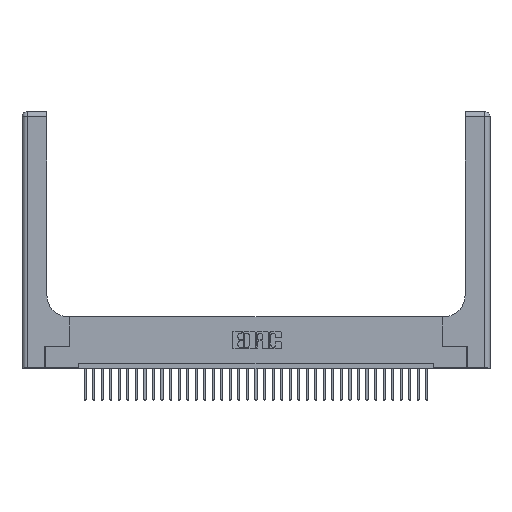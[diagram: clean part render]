
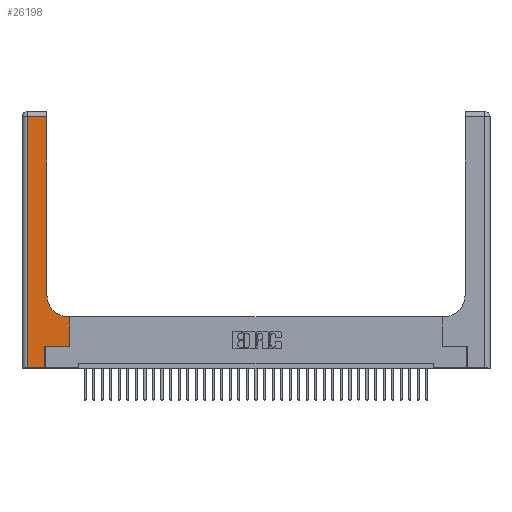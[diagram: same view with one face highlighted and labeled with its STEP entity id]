
A CAD part, top view. The second image highlights one B-rep face of the part: STEP entity #26198.
In plain terms, the highlighted planar face has unit normal (0, 0, 1).
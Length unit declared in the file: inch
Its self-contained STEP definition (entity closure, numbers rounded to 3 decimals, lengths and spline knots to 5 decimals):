
#583 = EDGE_CURVE ( 'NONE', #14601, #16200, #6018, .T. ) ;
#840 = CARTESIAN_POINT ( 'NONE',  ( 0.5585, 0.6, 0.37 ) ) ;
#1025 = DIRECTION ( 'NONE',  ( -1., 0., 0. ) ) ;
#1134 = CARTESIAN_POINT ( 'NONE',  ( 0.269, 0., 0.37 ) ) ;
#1947 = CIRCLE ( 'NONE', #6414, 0.25 ) ;
#1980 = LINE ( 'NONE', #19716, #35661 ) ;
#2318 = CARTESIAN_POINT ( 'NONE',  ( 0.06, 2.94, 0.37 ) ) ;
#2883 = DIRECTION ( 'NONE',  ( 1., 0., 0. ) ) ;
#3247 = ORIENTED_EDGE ( 'NONE', *, *, #31502, .T. ) ;
#3248 = VERTEX_POINT ( 'NONE', #18305 ) ;
#4439 = LINE ( 'NONE', #34091, #11006 ) ;
#4556 = DIRECTION ( 'NONE',  ( 1., 0., 0. ) ) ;
#5342 = VERTEX_POINT ( 'NONE', #9068 ) ;
#6018 = LINE ( 'NONE', #27974, #23095 ) ;
#6247 = EDGE_CURVE ( 'NONE', #16200, #3248, #16353, .T. ) ;
#6414 = AXIS2_PLACEMENT_3D ( 'NONE', #30180, #16047, #21751 ) ;
#6669 = CARTESIAN_POINT ( 'NONE',  ( 0.2915, 3., 0.37 ) ) ;
#7341 = LINE ( 'NONE', #6669, #21810 ) ;
#7647 = ORIENTED_EDGE ( 'NONE', *, *, #14574, .T. ) ;
#8733 = VERTEX_POINT ( 'NONE', #18860 ) ;
#9068 = CARTESIAN_POINT ( 'NONE',  ( 0.5415, 0.6, 0.37 ) ) ;
#9907 = ORIENTED_EDGE ( 'NONE', *, *, #32050, .T. ) ;
#10061 = CARTESIAN_POINT ( 'NONE',  ( 0.06, 3., 0.37 ) ) ;
#10184 = CARTESIAN_POINT ( 'NONE',  ( 0.269, 0.25, 0.37 ) ) ;
#10633 = CARTESIAN_POINT ( 'NONE',  ( 0.269, 0., 0.37 ) ) ;
#11006 = VECTOR ( 'NONE', #25754, 39.37008 ) ;
#11677 = CARTESIAN_POINT ( 'NONE',  ( 0.2915, 2.94, 0.37 ) ) ;
#11682 = EDGE_CURVE ( 'NONE', #3248, #31371, #22265, .T. ) ;
#12402 = LINE ( 'NONE', #17424, #30776 ) ;
#14312 = PLANE ( 'NONE',  #20672 ) ;
#14538 = VECTOR ( 'NONE', #27490, 39.37008 ) ;
#14574 = EDGE_CURVE ( 'NONE', #28070, #32074, #12402, .T. ) ;
#14601 = VERTEX_POINT ( 'NONE', #30248 ) ;
#16047 = DIRECTION ( 'NONE',  ( 0., 0., -1. ) ) ;
#16200 = VERTEX_POINT ( 'NONE', #1134 ) ;
#16353 = LINE ( 'NONE', #10633, #14538 ) ;
#17007 = CARTESIAN_POINT ( 'NONE',  ( 0., 3., 0.37 ) ) ;
#17248 = DIRECTION ( 'NONE',  ( 0., 0., -1. ) ) ;
#17424 = CARTESIAN_POINT ( 'NONE',  ( 0., 2.94, 0.37 ) ) ;
#18305 = CARTESIAN_POINT ( 'NONE',  ( 0.269, 0.25, 0.37 ) ) ;
#18860 = CARTESIAN_POINT ( 'NONE',  ( 0.2915, 0.85, 0.37 ) ) ;
#19140 = DIRECTION ( 'NONE',  ( 0., -1., 0. ) ) ;
#19222 = ORIENTED_EDGE ( 'NONE', *, *, #24231, .T. ) ;
#19716 = CARTESIAN_POINT ( 'NONE',  ( 0.5585, 0.25, 0.37 ) ) ;
#20672 = AXIS2_PLACEMENT_3D ( 'NONE', #17007, #17248, #33846 ) ;
#21419 = ORIENTED_EDGE ( 'NONE', *, *, #25837, .T. ) ;
#21751 = DIRECTION ( 'NONE',  ( 1., 0., 0. ) ) ;
#21810 = VECTOR ( 'NONE', #26244, 39.37008 ) ;
#22215 = LINE ( 'NONE', #10061, #35371 ) ;
#22265 = LINE ( 'NONE', #10184, #35421 ) ;
#22541 = VERTEX_POINT ( 'NONE', #840 ) ;
#22850 = ORIENTED_EDGE ( 'NONE', *, *, #29544, .T. ) ;
#23095 = VECTOR ( 'NONE', #2883, 39.37008 ) ;
#23939 = EDGE_LOOP ( 'NONE', ( #22850, #7647, #21419, #33977, #34716, #28946, #3247, #19222, #9907 ) ) ;
#24231 = EDGE_CURVE ( 'NONE', #22541, #5342, #4439, .T. ) ;
#25754 = DIRECTION ( 'NONE',  ( -1., 0., 0. ) ) ;
#25837 = EDGE_CURVE ( 'NONE', #32074, #14601, #22215, .T. ) ;
#26198 = ADVANCED_FACE ( 'NONE', ( #27421 ), #14312, .F. ) ;
#26244 = DIRECTION ( 'NONE',  ( 0., 1., 0. ) ) ;
#27421 = FACE_OUTER_BOUND ( 'NONE', #23939, .T. ) ;
#27490 = DIRECTION ( 'NONE',  ( 0., 1., 0. ) ) ;
#27646 = DIRECTION ( 'NONE',  ( 0., 1., 0. ) ) ;
#27974 = CARTESIAN_POINT ( 'NONE',  ( 0., 0., 0.37 ) ) ;
#28070 = VERTEX_POINT ( 'NONE', #11677 ) ;
#28946 = ORIENTED_EDGE ( 'NONE', *, *, #11682, .T. ) ;
#29544 = EDGE_CURVE ( 'NONE', #8733, #28070, #7341, .T. ) ;
#29866 = CARTESIAN_POINT ( 'NONE',  ( 0.5585, 0.25, 0.37 ) ) ;
#30180 = CARTESIAN_POINT ( 'NONE',  ( 0.5415, 0.85, 0.37 ) ) ;
#30248 = CARTESIAN_POINT ( 'NONE',  ( 0.06, 0., 0.37 ) ) ;
#30776 = VECTOR ( 'NONE', #1025, 39.37008 ) ;
#31371 = VERTEX_POINT ( 'NONE', #29866 ) ;
#31502 = EDGE_CURVE ( 'NONE', #31371, #22541, #1980, .T. ) ;
#32050 = EDGE_CURVE ( 'NONE', #5342, #8733, #1947, .T. ) ;
#32074 = VERTEX_POINT ( 'NONE', #2318 ) ;
#33846 = DIRECTION ( 'NONE',  ( -1., 0., 0. ) ) ;
#33977 = ORIENTED_EDGE ( 'NONE', *, *, #583, .T. ) ;
#34091 = CARTESIAN_POINT ( 'NONE',  ( 0.2915, 0.6, 0.37 ) ) ;
#34716 = ORIENTED_EDGE ( 'NONE', *, *, #6247, .T. ) ;
#35371 = VECTOR ( 'NONE', #19140, 39.37008 ) ;
#35421 = VECTOR ( 'NONE', #4556, 39.37008 ) ;
#35661 = VECTOR ( 'NONE', #27646, 39.37008 ) ;
